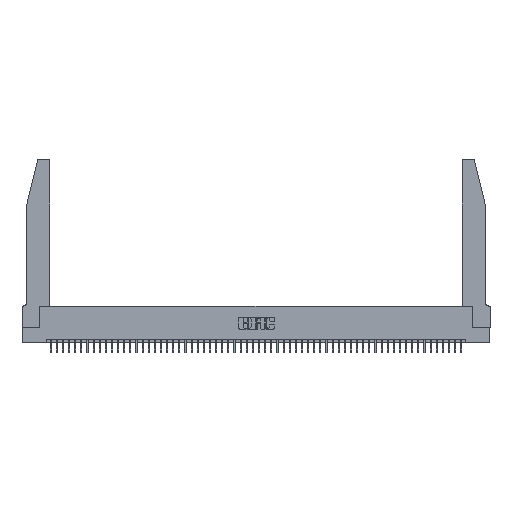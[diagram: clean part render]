
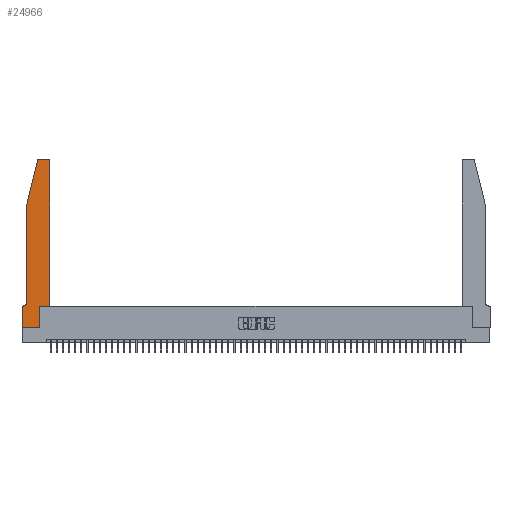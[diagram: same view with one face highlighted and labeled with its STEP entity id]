
A CAD part, top view. The second image highlights one B-rep face of the part: STEP entity #24966.
In plain terms, the highlighted planar face has unit normal (0, 0, 1).
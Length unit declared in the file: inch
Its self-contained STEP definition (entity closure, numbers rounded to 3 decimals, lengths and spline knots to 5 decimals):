
#507 = DIRECTION ( 'NONE',  ( 0., -1., 0. ) ) ;
#816 = ORIENTED_EDGE ( 'NONE', *, *, #43085, .T. ) ;
#901 = CARTESIAN_POINT ( 'NONE',  ( 0.284, 2.72, 0.37 ) ) ;
#931 = CIRCLE ( 'NONE', #38788, 0.03 ) ;
#1256 = VECTOR ( 'NONE', #507, 39.37008 ) ;
#1387 = LINE ( 'NONE', #49906, #10564 ) ;
#2757 = EDGE_CURVE ( 'NONE', #35166, #36234, #16875, .T. ) ;
#4550 = CARTESIAN_POINT ( 'NONE',  ( 0.0755, 2., 0.37 ) ) ;
#6408 = EDGE_CURVE ( 'NONE', #16085, #50032, #13810, .T. ) ;
#7395 = ORIENTED_EDGE ( 'NONE', *, *, #33398, .T. ) ;
#7526 = ORIENTED_EDGE ( 'NONE', *, *, #34476, .T. ) ;
#7631 = VECTOR ( 'NONE', #54301, 39.37008 ) ;
#8023 = VECTOR ( 'NONE', #13134, 39.37008 ) ;
#8290 = CARTESIAN_POINT ( 'NONE',  ( 0.4505, 0.35, 0.37 ) ) ;
#9362 = DIRECTION ( 'NONE',  ( 1., 0., 0. ) ) ;
#9646 = DIRECTION ( 'NONE',  ( -1., 0., 0. ) ) ;
#10399 = EDGE_CURVE ( 'NONE', #42823, #40089, #12469, .T. ) ;
#10564 = VECTOR ( 'NONE', #24255, 39.37008 ) ;
#11527 = CARTESIAN_POINT ( 'NONE',  ( 0.4505, 2.72, 0.37 ) ) ;
#12372 = ORIENTED_EDGE ( 'NONE', *, *, #28839, .T. ) ;
#12469 = LINE ( 'NONE', #17131, #27721 ) ;
#12517 = VERTEX_POINT ( 'NONE', #11527 ) ;
#13134 = DIRECTION ( 'NONE',  ( 1., 0., 0. ) ) ;
#13204 = AXIS2_PLACEMENT_3D ( 'NONE', #41993, #46208, #21255 ) ;
#13810 = LINE ( 'NONE', #4550, #1256 ) ;
#15638 = VECTOR ( 'NONE', #9646, 39.37008 ) ;
#16085 = VERTEX_POINT ( 'NONE', #39110 ) ;
#16087 = EDGE_CURVE ( 'NONE', #27309, #48504, #26946, .T. ) ;
#16295 = DIRECTION ( 'NONE',  ( 1., 0., 0. ) ) ;
#16875 = LINE ( 'NONE', #24923, #51306 ) ;
#17131 = CARTESIAN_POINT ( 'NONE',  ( 0.2605, 2.75, 0.37 ) ) ;
#17213 = CIRCLE ( 'NONE', #13204, 0.07 ) ;
#17740 = DIRECTION ( 'NONE',  ( 1., 0., 0. ) ) ;
#18153 = EDGE_LOOP ( 'NONE', ( #40286, #7395, #816, #45446, #12372, #41894, #23020, #27027, #51238, #7526, #34245, #33583 ) ) ;
#21255 = DIRECTION ( 'NONE',  ( -1., 0., 0. ) ) ;
#21325 = LINE ( 'NONE', #50293, #34017 ) ;
#22260 = CARTESIAN_POINT ( 'NONE',  ( 0.0755, 0.35, 0.37 ) ) ;
#22917 = LINE ( 'NONE', #8290, #7631 ) ;
#23020 = ORIENTED_EDGE ( 'NONE', *, *, #28707, .T. ) ;
#23265 = CARTESIAN_POINT ( 'NONE',  ( 0.0055, 0.35, 0.37 ) ) ;
#23756 = AXIS2_PLACEMENT_3D ( 'NONE', #41119, #28551, #16295 ) ;
#23813 = CARTESIAN_POINT ( 'NONE',  ( 0.0755, 0.42, 0.37 ) ) ;
#23974 = CARTESIAN_POINT ( 'NONE',  ( 0.284, 2.75, 0.37 ) ) ;
#24247 = CARTESIAN_POINT ( 'NONE',  ( 0., 0., 0.37 ) ) ;
#24255 = DIRECTION ( 'NONE',  ( 0., -1., 0. ) ) ;
#24330 = VECTOR ( 'NONE', #52526, 39.37008 ) ;
#24923 = CARTESIAN_POINT ( 'NONE',  ( 0.2865, 0.35, 0.37 ) ) ;
#24966 = ADVANCED_FACE ( 'NONE', ( #34265 ), #53782, .T. ) ;
#26224 = DIRECTION ( 'NONE',  ( -1., 0., 0. ) ) ;
#26946 = LINE ( 'NONE', #22260, #15638 ) ;
#27027 = ORIENTED_EDGE ( 'NONE', *, *, #46512, .T. ) ;
#27309 = VERTEX_POINT ( 'NONE', #23265 ) ;
#27632 = CARTESIAN_POINT ( 'NONE',  ( 0., 0., 0.37 ) ) ;
#27721 = VECTOR ( 'NONE', #26224, 39.37008 ) ;
#28551 = DIRECTION ( 'NONE',  ( 0., 0., 1. ) ) ;
#28707 = EDGE_CURVE ( 'NONE', #48504, #37594, #1387, .T. ) ;
#28839 = EDGE_CURVE ( 'NONE', #50032, #27309, #17213, .T. ) ;
#30757 = AXIS2_PLACEMENT_3D ( 'NONE', #901, #42497, #9362 ) ;
#31076 = CARTESIAN_POINT ( 'NONE',  ( 0.2865, 0.35, 0.37 ) ) ;
#33345 = CARTESIAN_POINT ( 'NONE',  ( 0., 0.35, 0.37 ) ) ;
#33398 = EDGE_CURVE ( 'NONE', #40089, #40644, #41293, .T. ) ;
#33583 = ORIENTED_EDGE ( 'NONE', *, *, #52905, .T. ) ;
#34017 = VECTOR ( 'NONE', #54145, 39.37008 ) ;
#34174 = VERTEX_POINT ( 'NONE', #48152 ) ;
#34245 = ORIENTED_EDGE ( 'NONE', *, *, #37838, .T. ) ;
#34252 = DIRECTION ( 'NONE',  ( 0., 0., 1. ) ) ;
#34265 = FACE_OUTER_BOUND ( 'NONE', #18153, .T. ) ;
#34476 = EDGE_CURVE ( 'NONE', #36234, #34174, #44473, .T. ) ;
#35166 = VERTEX_POINT ( 'NONE', #50408 ) ;
#36234 = VERTEX_POINT ( 'NONE', #31076 ) ;
#37594 = VERTEX_POINT ( 'NONE', #24247 ) ;
#37838 = EDGE_CURVE ( 'NONE', #34174, #12517, #22917, .T. ) ;
#38788 = AXIS2_PLACEMENT_3D ( 'NONE', #42910, #34252, #17740 ) ;
#39110 = CARTESIAN_POINT ( 'NONE',  ( 0.0755, 2., 0.37 ) ) ;
#40089 = VERTEX_POINT ( 'NONE', #23974 ) ;
#40286 = ORIENTED_EDGE ( 'NONE', *, *, #10399, .T. ) ;
#40644 = VERTEX_POINT ( 'NONE', #52364 ) ;
#41119 = CARTESIAN_POINT ( 'NONE',  ( 0., 0.35, 0.37 ) ) ;
#41211 = DIRECTION ( 'NONE',  ( 0., 1., 0. ) ) ;
#41293 = CIRCLE ( 'NONE', #30757, 0.03 ) ;
#41894 = ORIENTED_EDGE ( 'NONE', *, *, #16087, .T. ) ;
#41993 = CARTESIAN_POINT ( 'NONE',  ( 0.0055, 0.42, 0.37 ) ) ;
#42497 = DIRECTION ( 'NONE',  ( 0., 0., 1. ) ) ;
#42823 = VERTEX_POINT ( 'NONE', #47964 ) ;
#42910 = CARTESIAN_POINT ( 'NONE',  ( 0.4205, 2.72, 0.37 ) ) ;
#43085 = EDGE_CURVE ( 'NONE', #40644, #16085, #21325, .T. ) ;
#44473 = LINE ( 'NONE', #45690, #8023 ) ;
#45446 = ORIENTED_EDGE ( 'NONE', *, *, #6408, .T. ) ;
#45690 = CARTESIAN_POINT ( 'NONE',  ( 0.4505, 0.35, 0.37 ) ) ;
#46208 = DIRECTION ( 'NONE',  ( 0., 0., -1. ) ) ;
#46512 = EDGE_CURVE ( 'NONE', #37594, #35166, #48779, .T. ) ;
#47964 = CARTESIAN_POINT ( 'NONE',  ( 0.4205, 2.75, 0.37 ) ) ;
#48152 = CARTESIAN_POINT ( 'NONE',  ( 0.4505, 0.35, 0.37 ) ) ;
#48504 = VERTEX_POINT ( 'NONE', #33345 ) ;
#48779 = LINE ( 'NONE', #27632, #24330 ) ;
#49906 = CARTESIAN_POINT ( 'NONE',  ( 0., 0., 0.37 ) ) ;
#50032 = VERTEX_POINT ( 'NONE', #23813 ) ;
#50293 = CARTESIAN_POINT ( 'NONE',  ( 0.0755, 2., 0.37 ) ) ;
#50408 = CARTESIAN_POINT ( 'NONE',  ( 0.2865, 0., 0.37 ) ) ;
#51238 = ORIENTED_EDGE ( 'NONE', *, *, #2757, .T. ) ;
#51306 = VECTOR ( 'NONE', #41211, 39.37008 ) ;
#52364 = CARTESIAN_POINT ( 'NONE',  ( 0.25487, 2.72718, 0.37 ) ) ;
#52526 = DIRECTION ( 'NONE',  ( 1., 0., 0. ) ) ;
#52905 = EDGE_CURVE ( 'NONE', #12517, #42823, #931, .T. ) ;
#53782 = PLANE ( 'NONE',  #23756 ) ;
#54145 = DIRECTION ( 'NONE',  ( -0.239, -0.971, 0. ) ) ;
#54301 = DIRECTION ( 'NONE',  ( 0., 1., 0. ) ) ;
